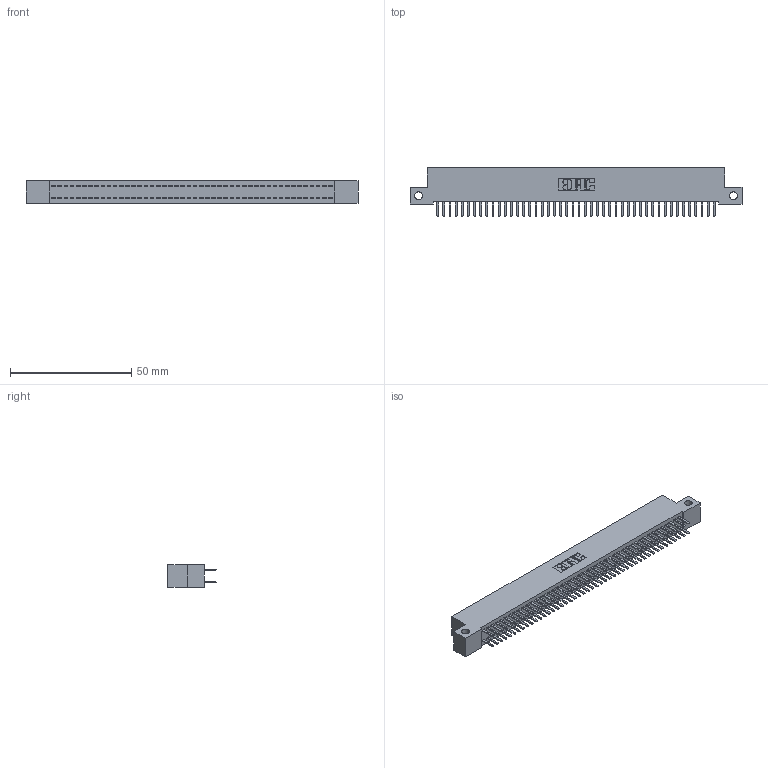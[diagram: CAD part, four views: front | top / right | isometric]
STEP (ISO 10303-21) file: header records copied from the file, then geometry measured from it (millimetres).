
FILE_DESCRIPTION (( 'STEP AP203' ), '1' );
FILE_NAME ('392-092-520-212.STEP', '2018-08-18T07:39:42', ( '' ), ( '' ), 'SwSTEP 2.0', 'SolidWorks 2016', '' );
FILE_SCHEMA (( 'CONFIG_CONTROL_DESIGN' ));
Length unit declared in the file: inch
Products named in the file (3): 342 Part_Side Mount; 345-292-001_345-293-120; 392-092-520-212
Assembly tree (93 placements, depth 2):
  392-092-520-212
    342 Part_Side Mount
    345-292-001_345-293-120  x92
Bounding box: 137.16 x 20.02 x 9.4 mm (x, y, z)
Volume: 12228.4 mm3; surface area: 19748.1 mm2
Topology: 93 solids, 93 shells, 5262 faces, 15295 edges, 9950 vertices
Faces by surface type: plane 3562, cylinder 1700
Entity records: 29061 total; most frequent: CARTESIAN_POINT 4822, ORIENTED_EDGE 4746, DIRECTION 4101, EDGE_CURVE 2373, VECTOR 2241, LINE 2241, VERTEX_POINT 1578, AXIS2_PLACEMENT_3D 930
